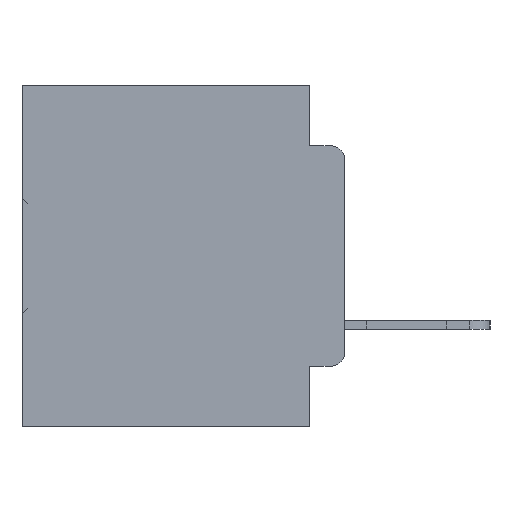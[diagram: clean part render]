
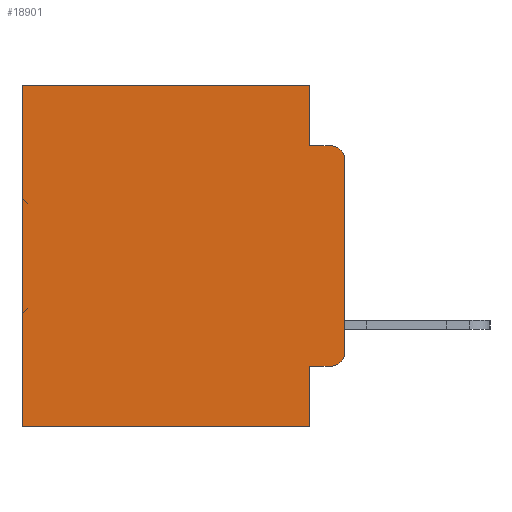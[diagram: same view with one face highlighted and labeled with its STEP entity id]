
A CAD part, left-side view. The second image highlights one B-rep face of the part: STEP entity #18901.
In plain terms, the highlighted planar face has unit normal (-1, 0, 0).
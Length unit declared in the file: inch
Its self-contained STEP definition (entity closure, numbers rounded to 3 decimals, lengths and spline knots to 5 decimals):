
#164 = AXIS2_PLACEMENT_3D ( 'NONE', #36282, #10991, #31993 ) ;
#245 = DIRECTION ( 'NONE',  ( 0., 1., 0. ) ) ;
#543 = CARTESIAN_POINT ( 'NONE',  ( 0.298, 0.473, 0. ) ) ;
#1498 = VERTEX_POINT ( 'NONE', #19761 ) ;
#1566 = CARTESIAN_POINT ( 'NONE',  ( 0.298, 0.051, -0.4115 ) ) ;
#2881 = CARTESIAN_POINT ( 'NONE',  ( 0.298, 0., -0.1085 ) ) ;
#3539 = VECTOR ( 'NONE', #18955, 39.37008 ) ;
#3759 = VECTOR ( 'NONE', #22825, 39.37008 ) ;
#6195 = EDGE_CURVE ( 'NONE', #24493, #10904, #31353, .T. ) ;
#6545 = ORIENTED_EDGE ( 'NONE', *, *, #6710, .T. ) ;
#6710 = EDGE_CURVE ( 'NONE', #30069, #27002, #7179, .T. ) ;
#6860 = CARTESIAN_POINT ( 'NONE',  ( 0.298, 0., -0.5 ) ) ;
#6900 = ORIENTED_EDGE ( 'NONE', *, *, #18416, .F. ) ;
#7179 = LINE ( 'NONE', #28822, #36301 ) ;
#7789 = DIRECTION ( 'NONE',  ( 0., -1., 0. ) ) ;
#8207 = EDGE_CURVE ( 'NONE', #28940, #10904, #25336, .T. ) ;
#9184 = AXIS2_PLACEMENT_3D ( 'NONE', #15104, #34576, #17982 ) ;
#9240 = ORIENTED_EDGE ( 'NONE', *, *, #20983, .F. ) ;
#10337 = VERTEX_POINT ( 'NONE', #28647 ) ;
#10344 = DIRECTION ( 'NONE',  ( 1., 0., 0. ) ) ;
#10904 = VERTEX_POINT ( 'NONE', #30871 ) ;
#10991 = DIRECTION ( 'NONE',  ( -1., 0., 0. ) ) ;
#11203 = CARTESIAN_POINT ( 'NONE',  ( 0.298, 0., 0. ) ) ;
#11680 = LINE ( 'NONE', #16134, #3539 ) ;
#12625 = ORIENTED_EDGE ( 'NONE', *, *, #8207, .F. ) ;
#13897 = CARTESIAN_POINT ( 'NONE',  ( 0.298, 0.051, 0. ) ) ;
#13959 = CARTESIAN_POINT ( 'NONE',  ( 0.298, 0.051, -0.4115 ) ) ;
#15070 = CARTESIAN_POINT ( 'NONE',  ( 0.298, 0.051, -0.0885 ) ) ;
#15104 = CARTESIAN_POINT ( 'NONE',  ( 0.298, 0.02, -0.3915 ) ) ;
#15370 = VECTOR ( 'NONE', #23501, 39.37008 ) ;
#15459 = ORIENTED_EDGE ( 'NONE', *, *, #34436, .T. ) ;
#15682 = CARTESIAN_POINT ( 'NONE',  ( 0.298, 0.051, -0.0885 ) ) ;
#16134 = CARTESIAN_POINT ( 'NONE',  ( 0.298, 0.051, 0. ) ) ;
#16883 = ORIENTED_EDGE ( 'NONE', *, *, #32646, .T. ) ;
#16983 = ORIENTED_EDGE ( 'NONE', *, *, #35479, .F. ) ;
#17705 = VECTOR ( 'NONE', #19922, 39.37008 ) ;
#17972 = ORIENTED_EDGE ( 'NONE', *, *, #6195, .T. ) ;
#17982 = DIRECTION ( 'NONE',  ( 0., 0., -1. ) ) ;
#18416 = EDGE_CURVE ( 'NONE', #25556, #10337, #22920, .T. ) ;
#18593 = LINE ( 'NONE', #543, #25215 ) ;
#18890 = ORIENTED_EDGE ( 'NONE', *, *, #33773, .T. ) ;
#18901 = ADVANCED_FACE ( 'NONE', ( #29488 ), #30319, .F. ) ;
#18955 = DIRECTION ( 'NONE',  ( 0., 0., -1. ) ) ;
#19146 = VECTOR ( 'NONE', #245, 39.37008 ) ;
#19576 = VECTOR ( 'NONE', #7789, 39.37008 ) ;
#19761 = CARTESIAN_POINT ( 'NONE',  ( 0.298, 0.473, -0.5 ) ) ;
#19922 = DIRECTION ( 'NONE',  ( 0., 0., -1. ) ) ;
#20983 = EDGE_CURVE ( 'NONE', #10337, #1498, #33905, .T. ) ;
#21607 = VERTEX_POINT ( 'NONE', #27250 ) ;
#21875 = CARTESIAN_POINT ( 'NONE',  ( 0.298, 0., 0. ) ) ;
#22825 = DIRECTION ( 'NONE',  ( 0., -1., 0. ) ) ;
#22920 = LINE ( 'NONE', #13897, #15370 ) ;
#23501 = DIRECTION ( 'NONE',  ( 0., 0., -1. ) ) ;
#24493 = VERTEX_POINT ( 'NONE', #2881 ) ;
#25215 = VECTOR ( 'NONE', #29943, 39.37008 ) ;
#25336 = LINE ( 'NONE', #15070, #3759 ) ;
#25556 = VERTEX_POINT ( 'NONE', #13959 ) ;
#26530 = AXIS2_PLACEMENT_3D ( 'NONE', #21875, #10344, #27610 ) ;
#27002 = VERTEX_POINT ( 'NONE', #33350 ) ;
#27250 = CARTESIAN_POINT ( 'NONE',  ( 0.298, 0.02, -0.4115 ) ) ;
#27610 = DIRECTION ( 'NONE',  ( 0., 0., -1. ) ) ;
#28647 = CARTESIAN_POINT ( 'NONE',  ( 0.298, 0.051, -0.5 ) ) ;
#28685 = ORIENTED_EDGE ( 'NONE', *, *, #37102, .F. ) ;
#28822 = CARTESIAN_POINT ( 'NONE',  ( 0.298, 0., 0. ) ) ;
#28940 = VERTEX_POINT ( 'NONE', #15682 ) ;
#29063 = DIRECTION ( 'NONE',  ( 0., 1., 0. ) ) ;
#29321 = VERTEX_POINT ( 'NONE', #31258 ) ;
#29488 = FACE_OUTER_BOUND ( 'NONE', #32926, .T. ) ;
#29943 = DIRECTION ( 'NONE',  ( 0., 0., -1. ) ) ;
#30069 = VERTEX_POINT ( 'NONE', #36601 ) ;
#30319 = PLANE ( 'NONE',  #26530 ) ;
#30871 = CARTESIAN_POINT ( 'NONE',  ( 0.298, 0.02, -0.0885 ) ) ;
#31258 = CARTESIAN_POINT ( 'NONE',  ( 0.298, 0., -0.3915 ) ) ;
#31353 = CIRCLE ( 'NONE', #164, 0.02 ) ;
#31993 = DIRECTION ( 'NONE',  ( 0., 0., -1. ) ) ;
#32646 = EDGE_CURVE ( 'NONE', #25556, #21607, #34340, .T. ) ;
#32926 = EDGE_LOOP ( 'NONE', ( #28685, #17972, #12625, #16983, #6545, #18890, #9240, #6900, #16883, #15459 ) ) ;
#33350 = CARTESIAN_POINT ( 'NONE',  ( 0.298, 0.473, 0. ) ) ;
#33773 = EDGE_CURVE ( 'NONE', #27002, #1498, #18593, .T. ) ;
#33905 = LINE ( 'NONE', #6860, #19146 ) ;
#34198 = LINE ( 'NONE', #11203, #17705 ) ;
#34340 = LINE ( 'NONE', #1566, #19576 ) ;
#34436 = EDGE_CURVE ( 'NONE', #21607, #29321, #36103, .T. ) ;
#34576 = DIRECTION ( 'NONE',  ( -1., 0., 0. ) ) ;
#35479 = EDGE_CURVE ( 'NONE', #30069, #28940, #11680, .T. ) ;
#36103 = CIRCLE ( 'NONE', #9184, 0.02 ) ;
#36282 = CARTESIAN_POINT ( 'NONE',  ( 0.298, 0.02, -0.1085 ) ) ;
#36301 = VECTOR ( 'NONE', #29063, 39.37008 ) ;
#36601 = CARTESIAN_POINT ( 'NONE',  ( 0.298, 0.051, 0. ) ) ;
#37102 = EDGE_CURVE ( 'NONE', #24493, #29321, #34198, .T. ) ;
